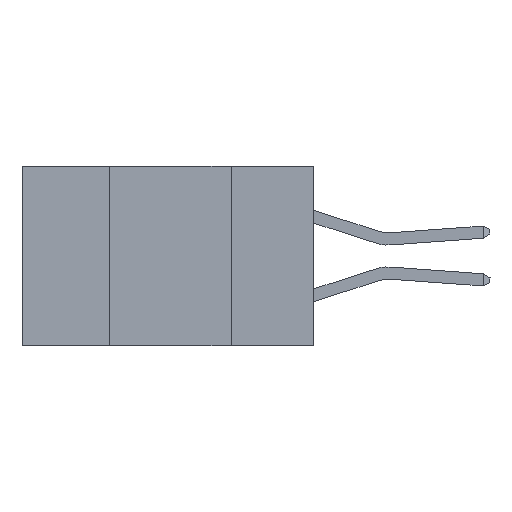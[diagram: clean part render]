
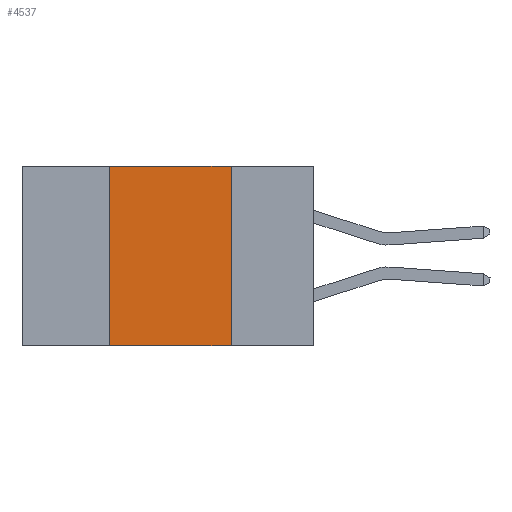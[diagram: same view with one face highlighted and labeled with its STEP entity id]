
A CAD part, left-side view. The second image highlights one B-rep face of the part: STEP entity #4537.
In plain terms, the highlighted planar face has unit normal (-1, 0, 0).
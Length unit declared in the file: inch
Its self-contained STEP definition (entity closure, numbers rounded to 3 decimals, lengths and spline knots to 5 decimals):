
#463 = DIRECTION ( 'NONE',  ( 0., -1., 0. ) ) ;
#1316 = CARTESIAN_POINT ( 'NONE',  ( 0., 0.42, 0. ) ) ;
#1481 = ORIENTED_EDGE ( 'NONE', *, *, #8015, .F. ) ;
#2051 = CARTESIAN_POINT ( 'NONE',  ( 0., 0.6, -0.37 ) ) ;
#2482 = CARTESIAN_POINT ( 'NONE',  ( 0., 0.17, 0. ) ) ;
#2712 = ORIENTED_EDGE ( 'NONE', *, *, #17033, .F. ) ;
#3290 = CARTESIAN_POINT ( 'NONE',  ( 0., 0.42, -0.37 ) ) ;
#3755 = LINE ( 'NONE', #2482, #12282 ) ;
#4037 = VECTOR ( 'NONE', #463, 39.37008 ) ;
#4537 = ADVANCED_FACE ( 'NONE', ( #16165 ), #12395, .F. ) ;
#5547 = CARTESIAN_POINT ( 'NONE',  ( 0., 0.17, -0.37 ) ) ;
#5715 = CARTESIAN_POINT ( 'NONE',  ( 0., 0.6, 0. ) ) ;
#7462 = DIRECTION ( 'NONE',  ( 0., 0., -1. ) ) ;
#8015 = EDGE_CURVE ( 'NONE', #16600, #19004, #13603, .T. ) ;
#8722 = CARTESIAN_POINT ( 'NONE',  ( 0., 0.17, 0. ) ) ;
#8755 = EDGE_CURVE ( 'NONE', #12390, #14116, #18995, .T. ) ;
#9483 = ORIENTED_EDGE ( 'NONE', *, *, #8755, .T. ) ;
#10218 = CARTESIAN_POINT ( 'NONE',  ( 0., 0.42, 0. ) ) ;
#10219 = VECTOR ( 'NONE', #15767, 39.37008 ) ;
#10274 = LINE ( 'NONE', #1316, #18533 ) ;
#10873 = EDGE_LOOP ( 'NONE', ( #2712, #1481, #19301, #9483 ) ) ;
#12282 = VECTOR ( 'NONE', #20997, 39.37008 ) ;
#12390 = VERTEX_POINT ( 'NONE', #3290 ) ;
#12395 = PLANE ( 'NONE',  #14114 ) ;
#13603 = LINE ( 'NONE', #20860, #4037 ) ;
#14114 = AXIS2_PLACEMENT_3D ( 'NONE', #5715, #17384, #7462 ) ;
#14116 = VERTEX_POINT ( 'NONE', #5547 ) ;
#15688 = EDGE_CURVE ( 'NONE', #12390, #16600, #10274, .T. ) ;
#15767 = DIRECTION ( 'NONE',  ( 0., -1., 0. ) ) ;
#16165 = FACE_OUTER_BOUND ( 'NONE', #10873, .T. ) ;
#16600 = VERTEX_POINT ( 'NONE', #10218 ) ;
#16761 = DIRECTION ( 'NONE',  ( 0., 0., 1. ) ) ;
#17033 = EDGE_CURVE ( 'NONE', #19004, #14116, #3755, .T. ) ;
#17384 = DIRECTION ( 'NONE',  ( 1., 0., 0. ) ) ;
#18533 = VECTOR ( 'NONE', #16761, 39.37008 ) ;
#18995 = LINE ( 'NONE', #2051, #10219 ) ;
#19004 = VERTEX_POINT ( 'NONE', #8722 ) ;
#19301 = ORIENTED_EDGE ( 'NONE', *, *, #15688, .F. ) ;
#20860 = CARTESIAN_POINT ( 'NONE',  ( 0., 0.6, 0. ) ) ;
#20997 = DIRECTION ( 'NONE',  ( 0., 0., -1. ) ) ;
